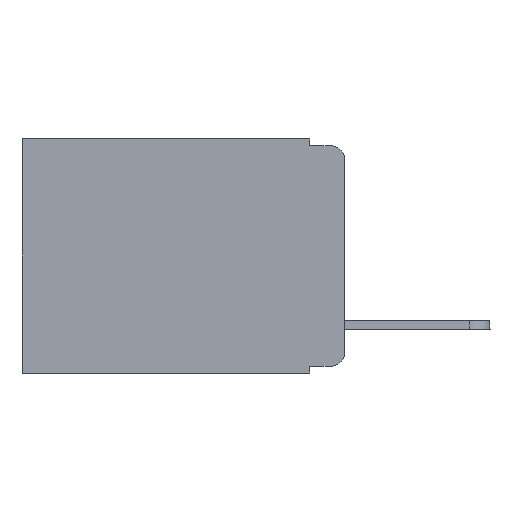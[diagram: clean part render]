
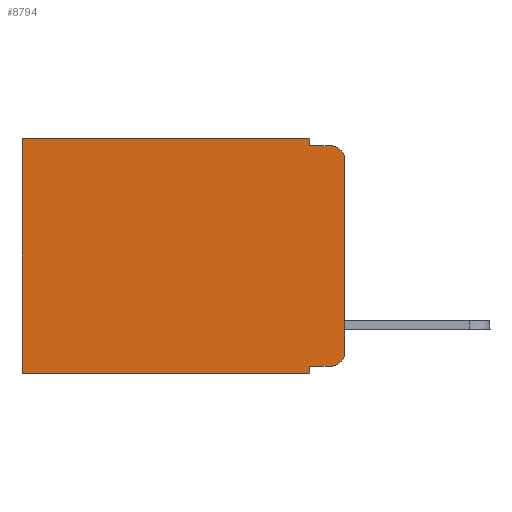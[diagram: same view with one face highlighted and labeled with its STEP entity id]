
A CAD part, left-side view. The second image highlights one B-rep face of the part: STEP entity #8794.
In plain terms, the highlighted planar face has unit normal (-1, 0, 0).
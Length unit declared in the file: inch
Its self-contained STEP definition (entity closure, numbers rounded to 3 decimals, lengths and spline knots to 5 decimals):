
#11 = LINE ( 'NONE', #21831, #3802 ) ;
#240 = DIRECTION ( 'NONE',  ( 0., 1., 0. ) ) ;
#465 = VECTOR ( 'NONE', #19301, 39.37008 ) ;
#645 = EDGE_LOOP ( 'NONE', ( #6765, #882, #16424, #22521, #13103, #25228, #13181, #10408, #21510, #3989 ) ) ;
#882 = ORIENTED_EDGE ( 'NONE', *, *, #1324, .T. ) ;
#1000 = EDGE_CURVE ( 'NONE', #23224, #22425, #23488, .T. ) ;
#1324 = EDGE_CURVE ( 'NONE', #24924, #12844, #12342, .T. ) ;
#1355 = DIRECTION ( 'NONE',  ( -1., 0., 0. ) ) ;
#1421 = CARTESIAN_POINT ( 'NONE',  ( 0.298, 0.051, -0.343 ) ) ;
#2238 = EDGE_CURVE ( 'NONE', #24924, #11632, #9759, .T. ) ;
#3603 = EDGE_CURVE ( 'NONE', #18145, #15698, #25405, .T. ) ;
#3658 = AXIS2_PLACEMENT_3D ( 'NONE', #11572, #1355, #9101 ) ;
#3802 = VECTOR ( 'NONE', #17580, 39.37008 ) ;
#3989 = ORIENTED_EDGE ( 'NONE', *, *, #13435, .T. ) ;
#4212 = CARTESIAN_POINT ( 'NONE',  ( 0.298, 0., 0. ) ) ;
#5122 = CARTESIAN_POINT ( 'NONE',  ( 0.298, 0., 0. ) ) ;
#5245 = FACE_OUTER_BOUND ( 'NONE', #645, .T. ) ;
#5302 = CARTESIAN_POINT ( 'NONE',  ( 0.298, 0.473, 0. ) ) ;
#5425 = AXIS2_PLACEMENT_3D ( 'NONE', #22690, #10971, #11226 ) ;
#5651 = CARTESIAN_POINT ( 'NONE',  ( 0.298, 0.473, 0. ) ) ;
#6765 = ORIENTED_EDGE ( 'NONE', *, *, #2238, .F. ) ;
#7114 = VECTOR ( 'NONE', #23076, 39.37008 ) ;
#8346 = DIRECTION ( 'NONE',  ( 0., 0., -1. ) ) ;
#8433 = VECTOR ( 'NONE', #240, 39.37008 ) ;
#8794 = ADVANCED_FACE ( 'NONE', ( #5245 ), #22823, .F. ) ;
#9101 = DIRECTION ( 'NONE',  ( 0., 0., -1. ) ) ;
#9537 = CARTESIAN_POINT ( 'NONE',  ( 0.298, 0.473, -0.343 ) ) ;
#9624 = VECTOR ( 'NONE', #14938, 39.37008 ) ;
#9759 = LINE ( 'NONE', #17631, #465 ) ;
#9917 = AXIS2_PLACEMENT_3D ( 'NONE', #5122, #11367, #20901 ) ;
#10408 = ORIENTED_EDGE ( 'NONE', *, *, #19176, .F. ) ;
#10645 = VERTEX_POINT ( 'NONE', #1421 ) ;
#10971 = DIRECTION ( 'NONE',  ( -1., 0., 0. ) ) ;
#11226 = DIRECTION ( 'NONE',  ( 0., 0., -1. ) ) ;
#11367 = DIRECTION ( 'NONE',  ( 1., 0., 0. ) ) ;
#11572 = CARTESIAN_POINT ( 'NONE',  ( 0.298, 0.02, -0.03 ) ) ;
#11632 = VERTEX_POINT ( 'NONE', #22240 ) ;
#11920 = CARTESIAN_POINT ( 'NONE',  ( 0.298, 0., -0.03 ) ) ;
#12342 = CIRCLE ( 'NONE', #3658, 0.02 ) ;
#12844 = VERTEX_POINT ( 'NONE', #14043 ) ;
#13103 = ORIENTED_EDGE ( 'NONE', *, *, #17744, .T. ) ;
#13159 = CARTESIAN_POINT ( 'NONE',  ( 0.298, 0.051, -0.333 ) ) ;
#13181 = ORIENTED_EDGE ( 'NONE', *, *, #22439, .F. ) ;
#13435 = EDGE_CURVE ( 'NONE', #24330, #11632, #24785, .T. ) ;
#13506 = VECTOR ( 'NONE', #8346, 39.37008 ) ;
#13743 = VECTOR ( 'NONE', #21139, 39.37008 ) ;
#14043 = CARTESIAN_POINT ( 'NONE',  ( 0.298, 0.02, -0.01 ) ) ;
#14816 = CARTESIAN_POINT ( 'NONE',  ( 0.298, 0.051, -0.333 ) ) ;
#14938 = DIRECTION ( 'NONE',  ( 0., -1., 0. ) ) ;
#15698 = VERTEX_POINT ( 'NONE', #17780 ) ;
#16424 = ORIENTED_EDGE ( 'NONE', *, *, #21723, .F. ) ;
#16491 = CARTESIAN_POINT ( 'NONE',  ( 0.298, 0.051, 0. ) ) ;
#17411 = LINE ( 'NONE', #25022, #7114 ) ;
#17580 = DIRECTION ( 'NONE',  ( 0., -1., 0. ) ) ;
#17631 = CARTESIAN_POINT ( 'NONE',  ( 0.298, 0., 0. ) ) ;
#17744 = EDGE_CURVE ( 'NONE', #18145, #23224, #21918, .T. ) ;
#17780 = CARTESIAN_POINT ( 'NONE',  ( 0.298, 0.051, -0.01 ) ) ;
#18145 = VERTEX_POINT ( 'NONE', #19819 ) ;
#19176 = EDGE_CURVE ( 'NONE', #22426, #10645, #24331, .T. ) ;
#19301 = DIRECTION ( 'NONE',  ( 0., 0., -1. ) ) ;
#19472 = CARTESIAN_POINT ( 'NONE',  ( 0.298, 0.051, 0. ) ) ;
#19819 = CARTESIAN_POINT ( 'NONE',  ( 0.298, 0.051, 0. ) ) ;
#20484 = DIRECTION ( 'NONE',  ( 0., 0., -1. ) ) ;
#20901 = DIRECTION ( 'NONE',  ( 0., 0., -1. ) ) ;
#21139 = DIRECTION ( 'NONE',  ( 0., 0., -1. ) ) ;
#21510 = ORIENTED_EDGE ( 'NONE', *, *, #22797, .T. ) ;
#21723 = EDGE_CURVE ( 'NONE', #15698, #12844, #11, .T. ) ;
#21831 = CARTESIAN_POINT ( 'NONE',  ( 0.298, 0.051, -0.01 ) ) ;
#21908 = VECTOR ( 'NONE', #20484, 39.37008 ) ;
#21918 = LINE ( 'NONE', #4212, #8433 ) ;
#22240 = CARTESIAN_POINT ( 'NONE',  ( 0.298, 0., -0.313 ) ) ;
#22425 = VERTEX_POINT ( 'NONE', #9537 ) ;
#22426 = VERTEX_POINT ( 'NONE', #13159 ) ;
#22439 = EDGE_CURVE ( 'NONE', #10645, #22425, #17411, .T. ) ;
#22521 = ORIENTED_EDGE ( 'NONE', *, *, #3603, .F. ) ;
#22690 = CARTESIAN_POINT ( 'NONE',  ( 0.298, 0.02, -0.313 ) ) ;
#22797 = EDGE_CURVE ( 'NONE', #22426, #24330, #23185, .T. ) ;
#22823 = PLANE ( 'NONE',  #9917 ) ;
#23076 = DIRECTION ( 'NONE',  ( 0., 1., 0. ) ) ;
#23185 = LINE ( 'NONE', #14816, #9624 ) ;
#23224 = VERTEX_POINT ( 'NONE', #5302 ) ;
#23488 = LINE ( 'NONE', #5651, #13506 ) ;
#24330 = VERTEX_POINT ( 'NONE', #24584 ) ;
#24331 = LINE ( 'NONE', #16491, #21908 ) ;
#24584 = CARTESIAN_POINT ( 'NONE',  ( 0.298, 0.02, -0.333 ) ) ;
#24785 = CIRCLE ( 'NONE', #5425, 0.02 ) ;
#24924 = VERTEX_POINT ( 'NONE', #11920 ) ;
#25022 = CARTESIAN_POINT ( 'NONE',  ( 0.298, 0., -0.343 ) ) ;
#25228 = ORIENTED_EDGE ( 'NONE', *, *, #1000, .T. ) ;
#25405 = LINE ( 'NONE', #19472, #13743 ) ;
